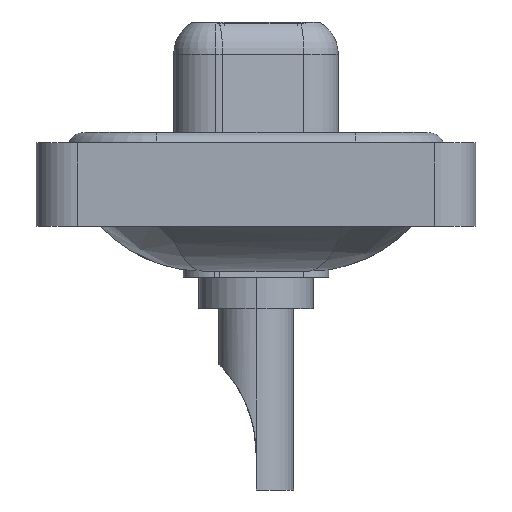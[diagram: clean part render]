
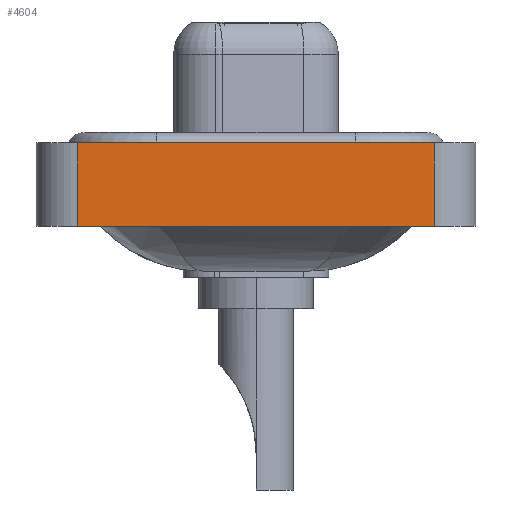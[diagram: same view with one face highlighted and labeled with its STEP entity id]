
A CAD part, left-side view. The second image highlights one B-rep face of the part: STEP entity #4604.
In plain terms, the highlighted planar face has unit normal (-1, 0, 0).
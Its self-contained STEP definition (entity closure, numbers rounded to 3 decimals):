
#949 = CARTESIAN_POINT ( 'NONE',  ( -7.25, 8.55, -3.6 ) ) ;
#1373 = VERTEX_POINT ( 'NONE', #10122 ) ;
#1801 = CARTESIAN_POINT ( 'NONE',  ( -7.25, -8.55, -3.6 ) ) ;
#1970 = LINE ( 'NONE', #1801, #16532 ) ;
#2728 = VECTOR ( 'NONE', #4447, 1000. ) ;
#3194 = VERTEX_POINT ( 'NONE', #16005 ) ;
#3476 = PLANE ( 'NONE',  #9017 ) ;
#3554 = DIRECTION ( 'NONE',  ( 0., -1., 0. ) ) ;
#4447 = DIRECTION ( 'NONE',  ( 0., 0., 1. ) ) ;
#4604 = ADVANCED_FACE ( 'NONE', ( #16380 ), #3476, .T. ) ;
#5015 = CARTESIAN_POINT ( 'NONE',  ( -7.25, 8.55, -3.6 ) ) ;
#5990 = LINE ( 'NONE', #5015, #10343 ) ;
#6109 = ORIENTED_EDGE ( 'NONE', *, *, #11280, .F. ) ;
#7165 = DIRECTION ( 'NONE',  ( 0., -1., 0. ) ) ;
#7365 = CARTESIAN_POINT ( 'NONE',  ( -7.25, -8.55, -3.6 ) ) ;
#8855 = DIRECTION ( 'NONE',  ( 0., 0., 1. ) ) ;
#9017 = AXIS2_PLACEMENT_3D ( 'NONE', #7365, #15070, #8855 ) ;
#9032 = LINE ( 'NONE', #11937, #10870 ) ;
#9058 = EDGE_LOOP ( 'NONE', ( #12745, #6109, #15312, #9122 ) ) ;
#9122 = ORIENTED_EDGE ( 'NONE', *, *, #10143, .T. ) ;
#9251 = VERTEX_POINT ( 'NONE', #949 ) ;
#10122 = CARTESIAN_POINT ( 'NONE',  ( -7.25, -8.55, -3.6 ) ) ;
#10132 = DIRECTION ( 'NONE',  ( 0., 0., 1. ) ) ;
#10143 = EDGE_CURVE ( 'NONE', #9251, #1373, #1970, .T. ) ;
#10343 = VECTOR ( 'NONE', #10132, 1000. ) ;
#10808 = EDGE_CURVE ( 'NONE', #9251, #12488, #5990, .T. ) ;
#10870 = VECTOR ( 'NONE', #3554, 1000. ) ;
#11280 = EDGE_CURVE ( 'NONE', #12488, #3194, #9032, .T. ) ;
#11937 = CARTESIAN_POINT ( 'NONE',  ( -7.25, -8.55, 0.4 ) ) ;
#12245 = EDGE_CURVE ( 'NONE', #1373, #3194, #15471, .T. ) ;
#12488 = VERTEX_POINT ( 'NONE', #15979 ) ;
#12745 = ORIENTED_EDGE ( 'NONE', *, *, #12245, .T. ) ;
#13892 = CARTESIAN_POINT ( 'NONE',  ( -7.25, -8.55, -3.6 ) ) ;
#15070 = DIRECTION ( 'NONE',  ( -1., 0., 0. ) ) ;
#15312 = ORIENTED_EDGE ( 'NONE', *, *, #10808, .F. ) ;
#15471 = LINE ( 'NONE', #13892, #2728 ) ;
#15979 = CARTESIAN_POINT ( 'NONE',  ( -7.25, 8.55, 0.4 ) ) ;
#16005 = CARTESIAN_POINT ( 'NONE',  ( -7.25, -8.55, 0.4 ) ) ;
#16380 = FACE_OUTER_BOUND ( 'NONE', #9058, .T. ) ;
#16532 = VECTOR ( 'NONE', #7165, 1000. ) ;
